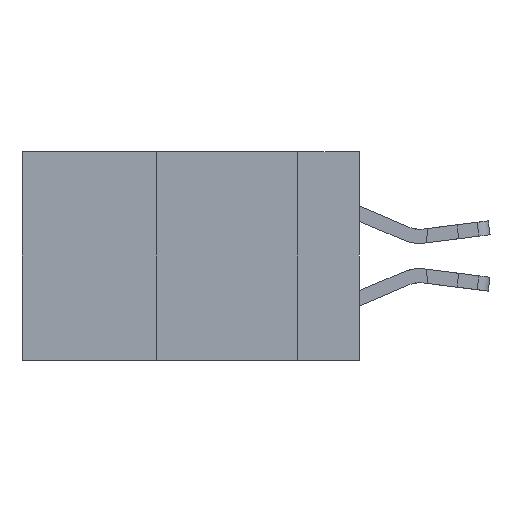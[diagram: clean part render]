
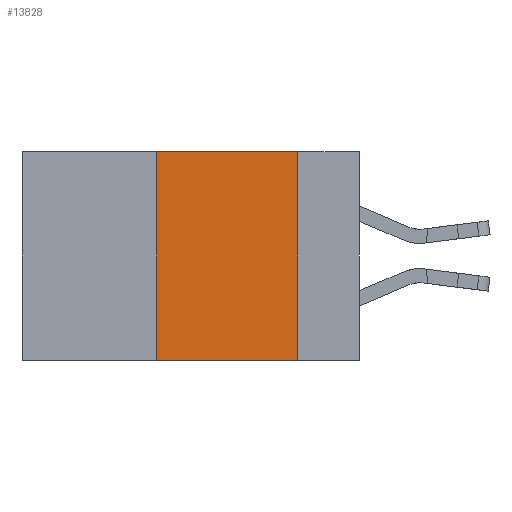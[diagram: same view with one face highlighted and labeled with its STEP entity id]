
A CAD part, left-side view. The second image highlights one B-rep face of the part: STEP entity #13828.
In plain terms, the highlighted planar face has unit normal (-1, 0, 0).
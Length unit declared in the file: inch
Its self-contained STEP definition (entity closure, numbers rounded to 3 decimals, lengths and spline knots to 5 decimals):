
#743 = LINE ( 'NONE', #9666, #7731 ) ;
#1191 = EDGE_LOOP ( 'NONE', ( #12478, #1984, #2732, #3181 ) ) ;
#1829 = DIRECTION ( 'NONE',  ( 0., 0., -1. ) ) ;
#1984 = ORIENTED_EDGE ( 'NONE', *, *, #9322, .F. ) ;
#2533 = CARTESIAN_POINT ( 'NONE',  ( 0., 0.36, 0. ) ) ;
#2732 = ORIENTED_EDGE ( 'NONE', *, *, #10764, .F. ) ;
#2884 = CARTESIAN_POINT ( 'NONE',  ( 0., 0.36, 0. ) ) ;
#3128 = CARTESIAN_POINT ( 'NONE',  ( 0., 0.6, 0. ) ) ;
#3181 = ORIENTED_EDGE ( 'NONE', *, *, #6431, .T. ) ;
#3455 = AXIS2_PLACEMENT_3D ( 'NONE', #5763, #14591, #7149 ) ;
#4355 = CARTESIAN_POINT ( 'NONE',  ( 0., 0.6, -0.37 ) ) ;
#4664 = FACE_OUTER_BOUND ( 'NONE', #1191, .T. ) ;
#4700 = LINE ( 'NONE', #4355, #11155 ) ;
#5511 = VECTOR ( 'NONE', #13341, 39.37008 ) ;
#5662 = DIRECTION ( 'NONE',  ( 0., -1., 0. ) ) ;
#5763 = CARTESIAN_POINT ( 'NONE',  ( 0., 0.6, 0. ) ) ;
#6431 = EDGE_CURVE ( 'NONE', #15251, #6653, #4700, .T. ) ;
#6504 = VECTOR ( 'NONE', #6838, 39.37008 ) ;
#6653 = VERTEX_POINT ( 'NONE', #14866 ) ;
#6838 = DIRECTION ( 'NONE',  ( 0., 0., 1. ) ) ;
#7149 = DIRECTION ( 'NONE',  ( 0., 0., -1. ) ) ;
#7731 = VECTOR ( 'NONE', #1829, 39.37008 ) ;
#9322 = EDGE_CURVE ( 'NONE', #11236, #16354, #15583, .T. ) ;
#9666 = CARTESIAN_POINT ( 'NONE',  ( 0., 0.11, 0. ) ) ;
#9975 = CARTESIAN_POINT ( 'NONE',  ( 0., 0.36, -0.37 ) ) ;
#10764 = EDGE_CURVE ( 'NONE', #15251, #11236, #16486, .T. ) ;
#11155 = VECTOR ( 'NONE', #5662, 39.37008 ) ;
#11236 = VERTEX_POINT ( 'NONE', #2533 ) ;
#11575 = EDGE_CURVE ( 'NONE', #16354, #6653, #743, .T. ) ;
#12478 = ORIENTED_EDGE ( 'NONE', *, *, #11575, .F. ) ;
#13341 = DIRECTION ( 'NONE',  ( 0., -1., 0. ) ) ;
#13369 = PLANE ( 'NONE',  #3455 ) ;
#13828 = ADVANCED_FACE ( 'NONE', ( #4664 ), #13369, .F. ) ;
#14591 = DIRECTION ( 'NONE',  ( 1., 0., 0. ) ) ;
#14866 = CARTESIAN_POINT ( 'NONE',  ( 0., 0.11, -0.37 ) ) ;
#15251 = VERTEX_POINT ( 'NONE', #9975 ) ;
#15398 = CARTESIAN_POINT ( 'NONE',  ( 0., 0.11, 0. ) ) ;
#15583 = LINE ( 'NONE', #3128, #5511 ) ;
#16354 = VERTEX_POINT ( 'NONE', #15398 ) ;
#16486 = LINE ( 'NONE', #2884, #6504 ) ;
